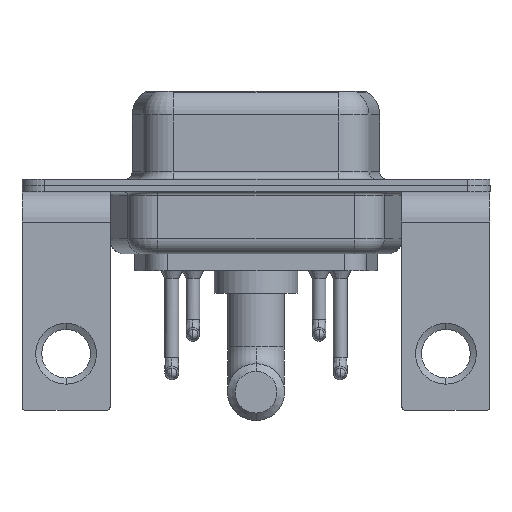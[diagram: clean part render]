
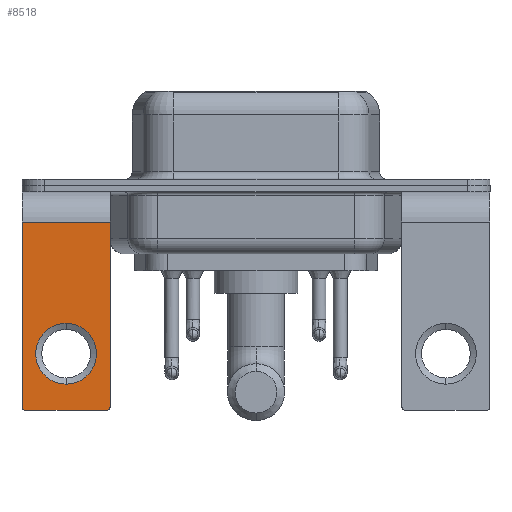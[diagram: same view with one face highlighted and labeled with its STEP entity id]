
A CAD part, front view. The second image highlights one B-rep face of the part: STEP entity #8518.
In plain terms, the highlighted planar face has unit normal (0, -1, 0).
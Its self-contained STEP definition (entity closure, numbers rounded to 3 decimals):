
#157 = EDGE_CURVE ( 'NONE', #2349, #1602, #7983, .T. ) ;
#286 = CARTESIAN_POINT ( 'NONE',  ( 2.9, -6.25, -14.55 ) ) ;
#320 = CARTESIAN_POINT ( 'NONE',  ( 2.9, -6.25, -2.4 ) ) ;
#422 = LINE ( 'NONE', #8488, #14368 ) ;
#615 = VECTOR ( 'NONE', #8104, 1000. ) ;
#927 = DIRECTION ( 'NONE',  ( 0., 1., 0. ) ) ;
#1043 = EDGE_LOOP ( 'NONE', ( #7891, #11724, #12223, #4622, #8556, #12802 ) ) ;
#1113 = DIRECTION ( 'NONE',  ( 0., 1., 0. ) ) ;
#1589 = VERTEX_POINT ( 'NONE', #5637 ) ;
#1602 = VERTEX_POINT ( 'NONE', #286 ) ;
#1688 = FACE_OUTER_BOUND ( 'NONE', #1043, .T. ) ;
#1723 = EDGE_CURVE ( 'NONE', #4387, #1602, #13976, .T. ) ;
#1778 = DIRECTION ( 'NONE',  ( 0., 0., 1. ) ) ;
#1988 = VERTEX_POINT ( 'NONE', #14551 ) ;
#2349 = VERTEX_POINT ( 'NONE', #5181 ) ;
#2401 = AXIS2_PLACEMENT_3D ( 'NONE', #320, #4372, #1778 ) ;
#3112 = CARTESIAN_POINT ( 'NONE',  ( 2.9, -6.25, -2.4 ) ) ;
#3476 = DIRECTION ( 'NONE',  ( 0., -1., 0. ) ) ;
#4178 = EDGE_CURVE ( 'NONE', #2349, #16275, #12372, .T. ) ;
#4372 = DIRECTION ( 'NONE',  ( 0., 1., 0. ) ) ;
#4387 = VERTEX_POINT ( 'NONE', #3112 ) ;
#4474 = VERTEX_POINT ( 'NONE', #5714 ) ;
#4622 = ORIENTED_EDGE ( 'NONE', *, *, #157, .T. ) ;
#5181 = CARTESIAN_POINT ( 'NONE',  ( 2.65, -6.25, -14.8 ) ) ;
#5634 = EDGE_CURVE ( 'NONE', #1988, #16275, #13951, .T. ) ;
#5637 = CARTESIAN_POINT ( 'NONE',  ( 0., -6.25, -9.07 ) ) ;
#5674 = FACE_BOUND ( 'NONE', #7807, .T. ) ;
#5714 = CARTESIAN_POINT ( 'NONE',  ( -2.9, -6.25, -2.4 ) ) ;
#6203 = AXIS2_PLACEMENT_3D ( 'NONE', #6541, #7840, #7749 ) ;
#6541 = CARTESIAN_POINT ( 'NONE',  ( -2.65, -6.25, -14.55 ) ) ;
#6963 = CIRCLE ( 'NONE', #11664, 2. ) ;
#7341 = CARTESIAN_POINT ( 'NONE',  ( 0., -6.25, -13.07 ) ) ;
#7719 = CIRCLE ( 'NONE', #7994, 2. ) ;
#7749 = DIRECTION ( 'NONE',  ( 0., 0., 1. ) ) ;
#7807 = EDGE_LOOP ( 'NONE', ( #10369, #9134 ) ) ;
#7840 = DIRECTION ( 'NONE',  ( 0., -1., 0. ) ) ;
#7891 = ORIENTED_EDGE ( 'NONE', *, *, #16678, .T. ) ;
#7983 = CIRCLE ( 'NONE', #16788, 0.25 ) ;
#7994 = AXIS2_PLACEMENT_3D ( 'NONE', #15633, #927, #14349 ) ;
#8104 = DIRECTION ( 'NONE',  ( -1., 0., 0. ) ) ;
#8488 = CARTESIAN_POINT ( 'NONE',  ( 2.9, -6.25, -2.4 ) ) ;
#8518 = ADVANCED_FACE ( 'NONE', ( #5674, #1688 ), #9676, .F. ) ;
#8556 = ORIENTED_EDGE ( 'NONE', *, *, #1723, .F. ) ;
#8856 = CARTESIAN_POINT ( 'NONE',  ( 2.65, -6.25, -14.55 ) ) ;
#9134 = ORIENTED_EDGE ( 'NONE', *, *, #14357, .T. ) ;
#9635 = LINE ( 'NONE', #13612, #13420 ) ;
#9676 = PLANE ( 'NONE',  #2401 ) ;
#9878 = VERTEX_POINT ( 'NONE', #7341 ) ;
#9907 = CARTESIAN_POINT ( 'NONE',  ( 2.9, -6.25, -2.4 ) ) ;
#10369 = ORIENTED_EDGE ( 'NONE', *, *, #11410, .T. ) ;
#10567 = DIRECTION ( 'NONE',  ( 0., 0., 1. ) ) ;
#10994 = DIRECTION ( 'NONE',  ( -1., 0., 0. ) ) ;
#11019 = DIRECTION ( 'NONE',  ( 0., 0., -1. ) ) ;
#11410 = EDGE_CURVE ( 'NONE', #9878, #1589, #7719, .T. ) ;
#11655 = VECTOR ( 'NONE', #15162, 1000. ) ;
#11664 = AXIS2_PLACEMENT_3D ( 'NONE', #13088, #1113, #10567 ) ;
#11724 = ORIENTED_EDGE ( 'NONE', *, *, #5634, .T. ) ;
#12223 = ORIENTED_EDGE ( 'NONE', *, *, #4178, .F. ) ;
#12252 = EDGE_CURVE ( 'NONE', #4387, #4474, #422, .T. ) ;
#12372 = LINE ( 'NONE', #13327, #615 ) ;
#12678 = DIRECTION ( 'NONE',  ( 0., 0., 1. ) ) ;
#12802 = ORIENTED_EDGE ( 'NONE', *, *, #12252, .T. ) ;
#13088 = CARTESIAN_POINT ( 'NONE',  ( 0., -6.25, -11.07 ) ) ;
#13327 = CARTESIAN_POINT ( 'NONE',  ( 2.9, -6.25, -14.8 ) ) ;
#13420 = VECTOR ( 'NONE', #11019, 1000. ) ;
#13490 = CARTESIAN_POINT ( 'NONE',  ( -2.65, -6.25, -14.8 ) ) ;
#13612 = CARTESIAN_POINT ( 'NONE',  ( -2.9, -6.25, -2.4 ) ) ;
#13951 = CIRCLE ( 'NONE', #6203, 0.25 ) ;
#13976 = LINE ( 'NONE', #9907, #11655 ) ;
#14349 = DIRECTION ( 'NONE',  ( 0., 0., 1. ) ) ;
#14357 = EDGE_CURVE ( 'NONE', #1589, #9878, #6963, .T. ) ;
#14368 = VECTOR ( 'NONE', #10994, 1000. ) ;
#14551 = CARTESIAN_POINT ( 'NONE',  ( -2.9, -6.25, -14.55 ) ) ;
#15162 = DIRECTION ( 'NONE',  ( 0., 0., -1. ) ) ;
#15633 = CARTESIAN_POINT ( 'NONE',  ( 0., -6.25, -11.07 ) ) ;
#16275 = VERTEX_POINT ( 'NONE', #13490 ) ;
#16678 = EDGE_CURVE ( 'NONE', #4474, #1988, #9635, .T. ) ;
#16788 = AXIS2_PLACEMENT_3D ( 'NONE', #8856, #3476, #12678 ) ;
